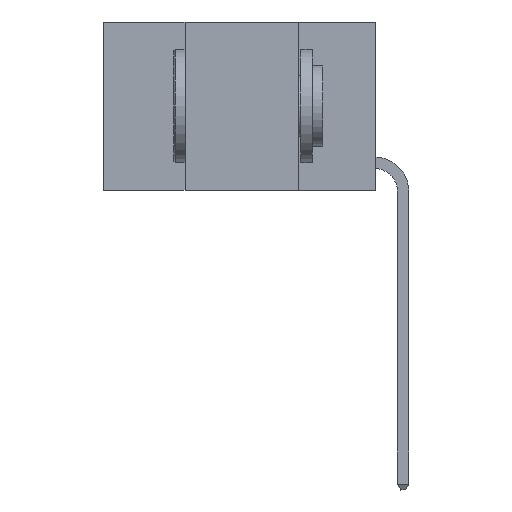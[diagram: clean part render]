
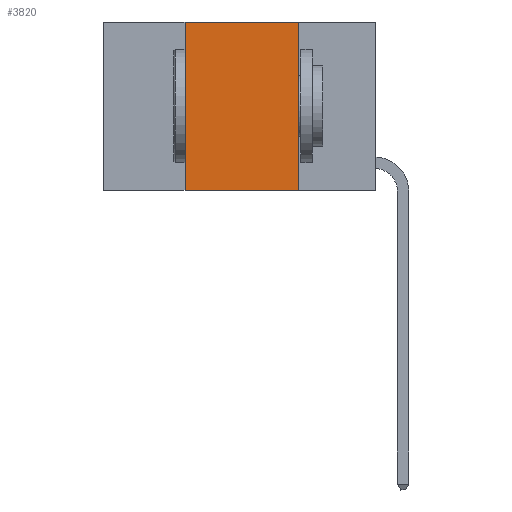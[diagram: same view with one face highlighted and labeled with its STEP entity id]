
A CAD part, left-side view. The second image highlights one B-rep face of the part: STEP entity #3820.
In plain terms, the highlighted planar face has unit normal (-1, 0, 0).
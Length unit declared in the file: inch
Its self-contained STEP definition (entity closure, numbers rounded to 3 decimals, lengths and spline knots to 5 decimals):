
#355 = EDGE_CURVE ( 'NONE', #4503, #20250, #19856, .T. ) ;
#568 = EDGE_CURVE ( 'NONE', #4503, #18114, #20218, .T. ) ;
#1140 = VECTOR ( 'NONE', #22239, 39.37008 ) ;
#2166 = CARTESIAN_POINT ( 'NONE',  ( 0., 0.42, 0. ) ) ;
#2173 = EDGE_CURVE ( 'NONE', #3732, #18114, #15024, .T. ) ;
#2205 = ORIENTED_EDGE ( 'NONE', *, *, #355, .F. ) ;
#2447 = CARTESIAN_POINT ( 'NONE',  ( 0., 0.17, 0. ) ) ;
#2554 = CARTESIAN_POINT ( 'NONE',  ( 0., 0.17, -0.37 ) ) ;
#3317 = EDGE_LOOP ( 'NONE', ( #3847, #7228, #2205, #18937 ) ) ;
#3732 = VERTEX_POINT ( 'NONE', #18606 ) ;
#3804 = VECTOR ( 'NONE', #17970, 39.37008 ) ;
#3820 = ADVANCED_FACE ( 'NONE', ( #19057 ), #15797, .F. ) ;
#3847 = ORIENTED_EDGE ( 'NONE', *, *, #2173, .F. ) ;
#4503 = VERTEX_POINT ( 'NONE', #13902 ) ;
#4628 = DIRECTION ( 'NONE',  ( 0., -1., 0. ) ) ;
#5508 = LINE ( 'NONE', #7363, #3804 ) ;
#7228 = ORIENTED_EDGE ( 'NONE', *, *, #18900, .F. ) ;
#7363 = CARTESIAN_POINT ( 'NONE',  ( 0., 0.6, 0. ) ) ;
#7495 = CARTESIAN_POINT ( 'NONE',  ( 0., 0.42, 0. ) ) ;
#7560 = DIRECTION ( 'NONE',  ( 0., 0., 1. ) ) ;
#8603 = CARTESIAN_POINT ( 'NONE',  ( 0., 0.6, 0. ) ) ;
#12336 = AXIS2_PLACEMENT_3D ( 'NONE', #8603, #17208, #17444 ) ;
#13708 = VECTOR ( 'NONE', #7560, 39.37008 ) ;
#13902 = CARTESIAN_POINT ( 'NONE',  ( 0., 0.42, -0.37 ) ) ;
#14845 = VECTOR ( 'NONE', #4628, 39.37008 ) ;
#15024 = LINE ( 'NONE', #2447, #1140 ) ;
#15797 = PLANE ( 'NONE',  #12336 ) ;
#17208 = DIRECTION ( 'NONE',  ( 1., 0., 0. ) ) ;
#17444 = DIRECTION ( 'NONE',  ( 0., 0., -1. ) ) ;
#17970 = DIRECTION ( 'NONE',  ( 0., -1., 0. ) ) ;
#18114 = VERTEX_POINT ( 'NONE', #2554 ) ;
#18606 = CARTESIAN_POINT ( 'NONE',  ( 0., 0.17, 0. ) ) ;
#18900 = EDGE_CURVE ( 'NONE', #20250, #3732, #5508, .T. ) ;
#18937 = ORIENTED_EDGE ( 'NONE', *, *, #568, .T. ) ;
#19057 = FACE_OUTER_BOUND ( 'NONE', #3317, .T. ) ;
#19856 = LINE ( 'NONE', #2166, #13708 ) ;
#20218 = LINE ( 'NONE', #22424, #14845 ) ;
#20250 = VERTEX_POINT ( 'NONE', #7495 ) ;
#22239 = DIRECTION ( 'NONE',  ( 0., 0., -1. ) ) ;
#22424 = CARTESIAN_POINT ( 'NONE',  ( 0., 0.6, -0.37 ) ) ;
